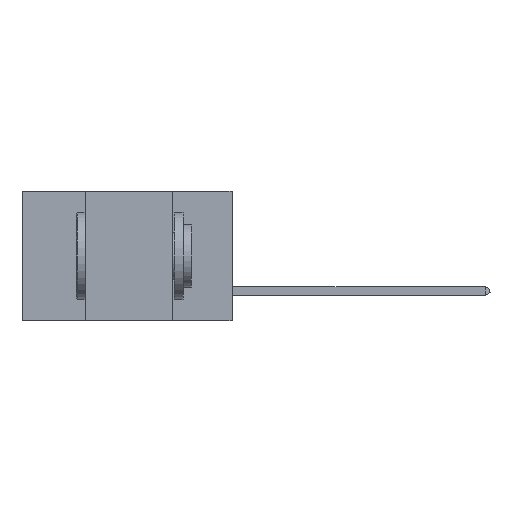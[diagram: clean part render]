
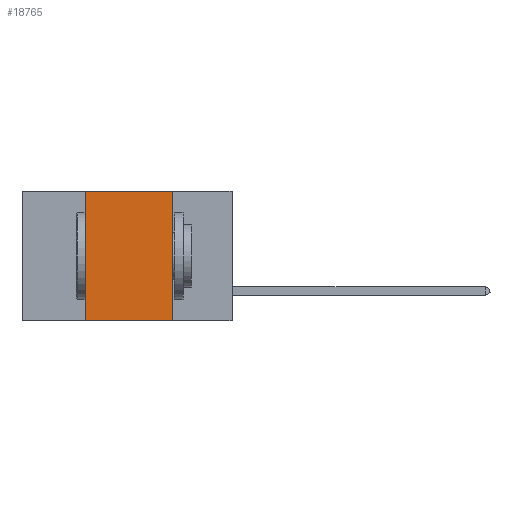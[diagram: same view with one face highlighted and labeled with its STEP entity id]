
A CAD part, left-side view. The second image highlights one B-rep face of the part: STEP entity #18765.
In plain terms, the highlighted planar face has unit normal (-1, 0, 0).
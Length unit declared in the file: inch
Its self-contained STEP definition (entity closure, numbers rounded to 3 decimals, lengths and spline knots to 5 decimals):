
#19 = ORIENTED_EDGE ( 'NONE', *, *, #11139, .F. ) ;
#781 = VERTEX_POINT ( 'NONE', #4325 ) ;
#1090 = CARTESIAN_POINT ( 'NONE',  ( 0., 0.42, 0. ) ) ;
#3179 = CARTESIAN_POINT ( 'NONE',  ( 0., 0.42, -0.37 ) ) ;
#3228 = LINE ( 'NONE', #9861, #13100 ) ;
#3513 = VERTEX_POINT ( 'NONE', #4837 ) ;
#3710 = DIRECTION ( 'NONE',  ( 0., -1., 0. ) ) ;
#4006 = LINE ( 'NONE', #21187, #8480 ) ;
#4119 = PLANE ( 'NONE',  #6442 ) ;
#4325 = CARTESIAN_POINT ( 'NONE',  ( 0., 0.17, 0. ) ) ;
#4350 = DIRECTION ( 'NONE',  ( 0., 0., 1. ) ) ;
#4837 = CARTESIAN_POINT ( 'NONE',  ( 0., 0.17, -0.37 ) ) ;
#6195 = DIRECTION ( 'NONE',  ( 0., 0., -1. ) ) ;
#6442 = AXIS2_PLACEMENT_3D ( 'NONE', #19235, #17629, #6195 ) ;
#7626 = DIRECTION ( 'NONE',  ( 0., -1., 0. ) ) ;
#8480 = VECTOR ( 'NONE', #7626, 39.37008 ) ;
#9052 = LINE ( 'NONE', #14560, #15053 ) ;
#9861 = CARTESIAN_POINT ( 'NONE',  ( 0., 0.42, 0. ) ) ;
#10808 = ORIENTED_EDGE ( 'NONE', *, *, #22787, .T. ) ;
#11139 = EDGE_CURVE ( 'NONE', #781, #3513, #9052, .T. ) ;
#11519 = LINE ( 'NONE', #15175, #16609 ) ;
#13100 = VECTOR ( 'NONE', #4350, 39.37008 ) ;
#13655 = ORIENTED_EDGE ( 'NONE', *, *, #14443, .F. ) ;
#14443 = EDGE_CURVE ( 'NONE', #18342, #781, #4006, .T. ) ;
#14560 = CARTESIAN_POINT ( 'NONE',  ( 0., 0.17, 0. ) ) ;
#14642 = DIRECTION ( 'NONE',  ( 0., 0., -1. ) ) ;
#15053 = VECTOR ( 'NONE', #14642, 39.37008 ) ;
#15175 = CARTESIAN_POINT ( 'NONE',  ( 0., 0.6, -0.37 ) ) ;
#16609 = VECTOR ( 'NONE', #3710, 39.37008 ) ;
#17629 = DIRECTION ( 'NONE',  ( 1., 0., 0. ) ) ;
#18342 = VERTEX_POINT ( 'NONE', #1090 ) ;
#18765 = ADVANCED_FACE ( 'NONE', ( #20887 ), #4119, .F. ) ;
#19235 = CARTESIAN_POINT ( 'NONE',  ( 0., 0.6, 0. ) ) ;
#19580 = VERTEX_POINT ( 'NONE', #3179 ) ;
#20270 = ORIENTED_EDGE ( 'NONE', *, *, #20570, .F. ) ;
#20570 = EDGE_CURVE ( 'NONE', #19580, #18342, #3228, .T. ) ;
#20887 = FACE_OUTER_BOUND ( 'NONE', #22658, .T. ) ;
#21187 = CARTESIAN_POINT ( 'NONE',  ( 0., 0.6, 0. ) ) ;
#22658 = EDGE_LOOP ( 'NONE', ( #19, #13655, #20270, #10808 ) ) ;
#22787 = EDGE_CURVE ( 'NONE', #19580, #3513, #11519, .T. ) ;
